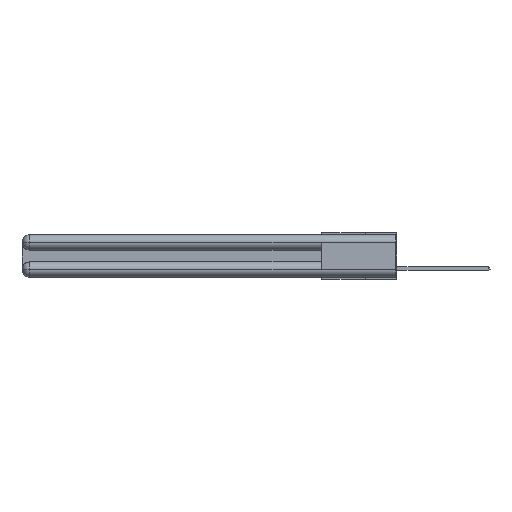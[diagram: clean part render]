
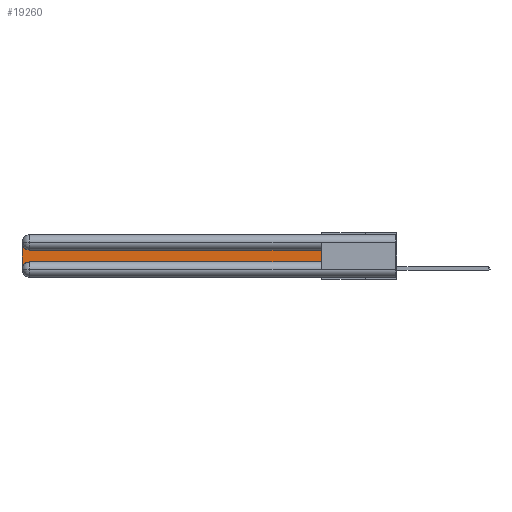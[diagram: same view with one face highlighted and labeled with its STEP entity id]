
A CAD part, left-side view. The second image highlights one B-rep face of the part: STEP entity #19260.
In plain terms, the highlighted planar face has unit normal (-1, 0, 0).
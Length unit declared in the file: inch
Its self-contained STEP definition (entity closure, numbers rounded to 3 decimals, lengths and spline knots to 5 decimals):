
#949 = VECTOR ( 'NONE', #14644, 39.37008 ) ;
#1943 = EDGE_LOOP ( 'NONE', ( #20582, #5579, #31017, #25897, #13260, #31945 ) ) ;
#2668 = VERTEX_POINT ( 'NONE', #19540 ) ;
#4043 = CARTESIAN_POINT ( 'NONE',  ( 0.075, 0.6, -0.2175 ) ) ;
#4283 = PLANE ( 'NONE',  #27327 ) ;
#4900 = CARTESIAN_POINT ( 'NONE',  ( 0.075, 0.6, -0.1225 ) ) ;
#5336 = DIRECTION ( 'NONE',  ( 1., 0., 0. ) ) ;
#5579 = ORIENTED_EDGE ( 'NONE', *, *, #20126, .T. ) ;
#7332 = VECTOR ( 'NONE', #27033, 39.37008 ) ;
#7828 = CIRCLE ( 'NONE', #15091, 0.06 ) ;
#8327 = EDGE_CURVE ( 'NONE', #31596, #29251, #28318, .T. ) ;
#9121 = CARTESIAN_POINT ( 'NONE',  ( 0.075, 3., -0.0625 ) ) ;
#9648 = DIRECTION ( 'NONE',  ( 0., 0., -1. ) ) ;
#9864 = VECTOR ( 'NONE', #29923, 39.37008 ) ;
#12863 = EDGE_CURVE ( 'NONE', #29251, #2668, #20236, .T. ) ;
#12965 = CIRCLE ( 'NONE', #25224, 0.06 ) ;
#13260 = ORIENTED_EDGE ( 'NONE', *, *, #8327, .T. ) ;
#13393 = EDGE_CURVE ( 'NONE', #28244, #31596, #12965, .T. ) ;
#14644 = DIRECTION ( 'NONE',  ( 0., 0., -1. ) ) ;
#15091 = AXIS2_PLACEMENT_3D ( 'NONE', #17546, #22623, #30323 ) ;
#17546 = CARTESIAN_POINT ( 'NONE',  ( 0.075, 2.94, -0.0625 ) ) ;
#18236 = CARTESIAN_POINT ( 'NONE',  ( 0.075, 2.94, -0.2775 ) ) ;
#18331 = FACE_OUTER_BOUND ( 'NONE', #1943, .T. ) ;
#19260 = ADVANCED_FACE ( 'NONE', ( #18331 ), #4283, .F. ) ;
#19540 = CARTESIAN_POINT ( 'NONE',  ( 0.075, 0.6, -0.1225 ) ) ;
#20053 = CARTESIAN_POINT ( 'NONE',  ( 0.075, 2.94, -0.2175 ) ) ;
#20126 = EDGE_CURVE ( 'NONE', #23101, #20640, #7828, .T. ) ;
#20236 = LINE ( 'NONE', #24688, #30261 ) ;
#20582 = ORIENTED_EDGE ( 'NONE', *, *, #24787, .T. ) ;
#20640 = VERTEX_POINT ( 'NONE', #9121 ) ;
#21094 = EDGE_CURVE ( 'NONE', #20640, #28244, #29844, .T. ) ;
#21880 = CARTESIAN_POINT ( 'NONE',  ( 0.075, 2.94, -0.1225 ) ) ;
#22311 = CARTESIAN_POINT ( 'NONE',  ( 0.075, 3., -0.2175 ) ) ;
#22575 = DIRECTION ( 'NONE',  ( 1., 0., 0. ) ) ;
#22623 = DIRECTION ( 'NONE',  ( 1., 0., 0. ) ) ;
#23101 = VERTEX_POINT ( 'NONE', #21880 ) ;
#23307 = DIRECTION ( 'NONE',  ( 0., 0., -1. ) ) ;
#24688 = CARTESIAN_POINT ( 'NONE',  ( 0.075, 0.6, -0.2175 ) ) ;
#24787 = EDGE_CURVE ( 'NONE', #2668, #23101, #27426, .T. ) ;
#25224 = AXIS2_PLACEMENT_3D ( 'NONE', #18236, #5336, #23307 ) ;
#25897 = ORIENTED_EDGE ( 'NONE', *, *, #13393, .T. ) ;
#27033 = DIRECTION ( 'NONE',  ( 0., 1., 0. ) ) ;
#27126 = DIRECTION ( 'NONE',  ( 0., 0., 1. ) ) ;
#27327 = AXIS2_PLACEMENT_3D ( 'NONE', #30058, #22575, #9648 ) ;
#27426 = LINE ( 'NONE', #4900, #7332 ) ;
#27673 = CARTESIAN_POINT ( 'NONE',  ( 0.075, 3., -0.2775 ) ) ;
#28244 = VERTEX_POINT ( 'NONE', #27673 ) ;
#28285 = CARTESIAN_POINT ( 'NONE',  ( 0.075, 0.6, -0.2175 ) ) ;
#28318 = LINE ( 'NONE', #4043, #9864 ) ;
#29251 = VERTEX_POINT ( 'NONE', #28285 ) ;
#29844 = LINE ( 'NONE', #22311, #949 ) ;
#29923 = DIRECTION ( 'NONE',  ( 0., -1., 0. ) ) ;
#30058 = CARTESIAN_POINT ( 'NONE',  ( 0.075, 3., -0.1225 ) ) ;
#30261 = VECTOR ( 'NONE', #27126, 39.37008 ) ;
#30323 = DIRECTION ( 'NONE',  ( 0., 0., -1. ) ) ;
#31017 = ORIENTED_EDGE ( 'NONE', *, *, #21094, .T. ) ;
#31596 = VERTEX_POINT ( 'NONE', #20053 ) ;
#31945 = ORIENTED_EDGE ( 'NONE', *, *, #12863, .T. ) ;
